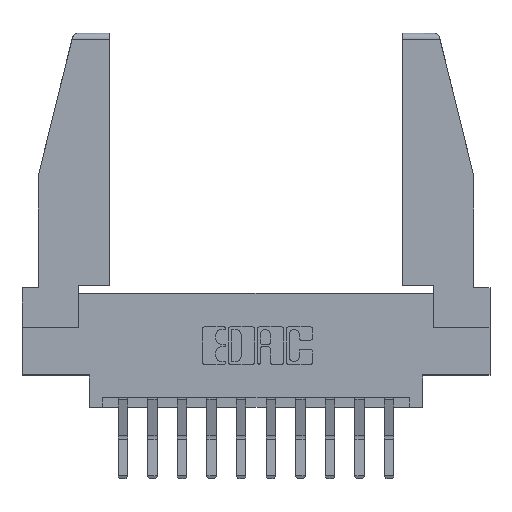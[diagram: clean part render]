
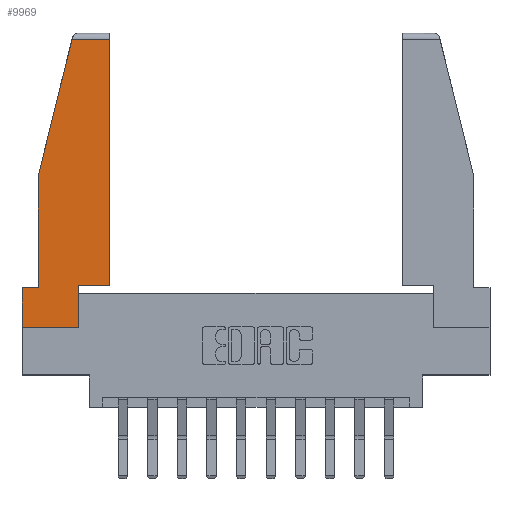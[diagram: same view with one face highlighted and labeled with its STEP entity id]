
A CAD part, top view. The second image highlights one B-rep face of the part: STEP entity #9969.
In plain terms, the highlighted planar face has unit normal (0, 0, 1).
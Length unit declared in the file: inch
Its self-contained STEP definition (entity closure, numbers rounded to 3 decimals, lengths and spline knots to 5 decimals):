
#61 = CARTESIAN_POINT ( 'NONE',  ( 0.271, 1.55, 0. ) ) ;
#64 = ORIENTED_EDGE ( 'NONE', *, *, #14433, .T. ) ;
#294 = VERTEX_POINT ( 'NONE', #4942 ) ;
#372 = ORIENTED_EDGE ( 'NONE', *, *, #10486, .T. ) ;
#478 = ORIENTED_EDGE ( 'NONE', *, *, #6683, .T. ) ;
#932 = FACE_OUTER_BOUND ( 'NONE', #4753, .T. ) ;
#1284 = LINE ( 'NONE', #9256, #14321 ) ;
#1523 = ORIENTED_EDGE ( 'NONE', *, *, #4932, .T. ) ;
#2094 = ORIENTED_EDGE ( 'NONE', *, *, #4949, .T. ) ;
#2324 = CARTESIAN_POINT ( 'NONE',  ( 0.086, 0.8, 0. ) ) ;
#2447 = LINE ( 'NONE', #4228, #11066 ) ;
#2624 = VERTEX_POINT ( 'NONE', #9388 ) ;
#2800 = VERTEX_POINT ( 'NONE', #11313 ) ;
#3058 = CARTESIAN_POINT ( 'NONE',  ( 0.297, 0.223, 0. ) ) ;
#3356 = DIRECTION ( 'NONE',  ( 1., 0., 0. ) ) ;
#3465 = CARTESIAN_POINT ( 'NONE',  ( 0., 0., 0. ) ) ;
#3572 = AXIS2_PLACEMENT_3D ( 'NONE', #6690, #7822, #3356 ) ;
#3856 = VECTOR ( 'NONE', #12459, 39.37008 ) ;
#4092 = DIRECTION ( 'NONE',  ( 0., 1., 0. ) ) ;
#4228 = CARTESIAN_POINT ( 'NONE',  ( 0., 0.21, 0. ) ) ;
#4248 = CARTESIAN_POINT ( 'NONE',  ( 0., 0.21, 0. ) ) ;
#4294 = EDGE_CURVE ( 'NONE', #7948, #10404, #14289, .T. ) ;
#4326 = DIRECTION ( 'NONE',  ( -0.239, -0.971, 0. ) ) ;
#4417 = PLANE ( 'NONE',  #3572 ) ;
#4753 = EDGE_LOOP ( 'NONE', ( #1523, #478, #9538, #10084, #7608, #64, #372, #14084, #2094 ) ) ;
#4932 = EDGE_CURVE ( 'NONE', #12422, #10001, #12996, .T. ) ;
#4942 = CARTESIAN_POINT ( 'NONE',  ( 0.297, 0., 0. ) ) ;
#4949 = EDGE_CURVE ( 'NONE', #9905, #12422, #5164, .T. ) ;
#5164 = LINE ( 'NONE', #13174, #9595 ) ;
#5518 = CARTESIAN_POINT ( 'NONE',  ( 0.086, 0.21, 0. ) ) ;
#5767 = CARTESIAN_POINT ( 'NONE',  ( 0.2636, 1.52, 0. ) ) ;
#6000 = LINE ( 'NONE', #61, #9358 ) ;
#6603 = VECTOR ( 'NONE', #6629, 39.37008 ) ;
#6629 = DIRECTION ( 'NONE',  ( -1., 0., 0. ) ) ;
#6683 = EDGE_CURVE ( 'NONE', #10001, #8061, #8301, .T. ) ;
#6690 = CARTESIAN_POINT ( 'NONE',  ( 0., 0., 0. ) ) ;
#6770 = VECTOR ( 'NONE', #4092, 39.37008 ) ;
#7131 = DIRECTION ( 'NONE',  ( -1., 0., 0. ) ) ;
#7210 = LINE ( 'NONE', #3465, #3856 ) ;
#7482 = EDGE_CURVE ( 'NONE', #10404, #2800, #8347, .T. ) ;
#7608 = ORIENTED_EDGE ( 'NONE', *, *, #7482, .T. ) ;
#7822 = DIRECTION ( 'NONE',  ( 0., 0., 1. ) ) ;
#7894 = VECTOR ( 'NONE', #11818, 39.37008 ) ;
#7948 = VERTEX_POINT ( 'NONE', #2324 ) ;
#8061 = VERTEX_POINT ( 'NONE', #5767 ) ;
#8301 = LINE ( 'NONE', #12859, #14540 ) ;
#8347 = LINE ( 'NONE', #4248, #6603 ) ;
#8381 = CARTESIAN_POINT ( 'NONE',  ( 0.086, 0.8, 0. ) ) ;
#9256 = CARTESIAN_POINT ( 'NONE',  ( 0.297, 0., 0. ) ) ;
#9358 = VECTOR ( 'NONE', #4326, 39.37008 ) ;
#9388 = CARTESIAN_POINT ( 'NONE',  ( 0., 0., 0. ) ) ;
#9538 = ORIENTED_EDGE ( 'NONE', *, *, #9555, .T. ) ;
#9555 = EDGE_CURVE ( 'NONE', #8061, #7948, #6000, .T. ) ;
#9595 = VECTOR ( 'NONE', #9922, 39.37008 ) ;
#9905 = VERTEX_POINT ( 'NONE', #3058 ) ;
#9922 = DIRECTION ( 'NONE',  ( 1., 0., 0. ) ) ;
#9969 = ADVANCED_FACE ( 'NONE', ( #932 ), #4417, .T. ) ;
#10001 = VERTEX_POINT ( 'NONE', #11407 ) ;
#10084 = ORIENTED_EDGE ( 'NONE', *, *, #4294, .T. ) ;
#10106 = EDGE_CURVE ( 'NONE', #294, #9905, #1284, .T. ) ;
#10401 = DIRECTION ( 'NONE',  ( 0., 1., 0. ) ) ;
#10404 = VERTEX_POINT ( 'NONE', #5518 ) ;
#10486 = EDGE_CURVE ( 'NONE', #2624, #294, #7210, .T. ) ;
#10878 = CARTESIAN_POINT ( 'NONE',  ( 0.461, 0.223, 0. ) ) ;
#11066 = VECTOR ( 'NONE', #13268, 39.37008 ) ;
#11313 = CARTESIAN_POINT ( 'NONE',  ( 0., 0.21, 0. ) ) ;
#11407 = CARTESIAN_POINT ( 'NONE',  ( 0.461, 1.52, 0. ) ) ;
#11818 = DIRECTION ( 'NONE',  ( 0., -1., 0. ) ) ;
#12334 = CARTESIAN_POINT ( 'NONE',  ( 0.461, 0.223, 0. ) ) ;
#12422 = VERTEX_POINT ( 'NONE', #12334 ) ;
#12459 = DIRECTION ( 'NONE',  ( 1., 0., 0. ) ) ;
#12859 = CARTESIAN_POINT ( 'NONE',  ( 0., 1.52, 0. ) ) ;
#12996 = LINE ( 'NONE', #10878, #6770 ) ;
#13174 = CARTESIAN_POINT ( 'NONE',  ( 0.297, 0.223, 0. ) ) ;
#13268 = DIRECTION ( 'NONE',  ( 0., -1., 0. ) ) ;
#14084 = ORIENTED_EDGE ( 'NONE', *, *, #10106, .T. ) ;
#14289 = LINE ( 'NONE', #8381, #7894 ) ;
#14321 = VECTOR ( 'NONE', #10401, 39.37008 ) ;
#14433 = EDGE_CURVE ( 'NONE', #2800, #2624, #2447, .T. ) ;
#14540 = VECTOR ( 'NONE', #7131, 39.37008 ) ;
